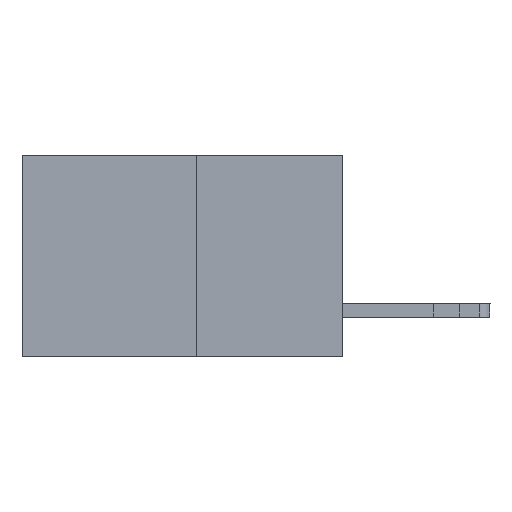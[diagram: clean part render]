
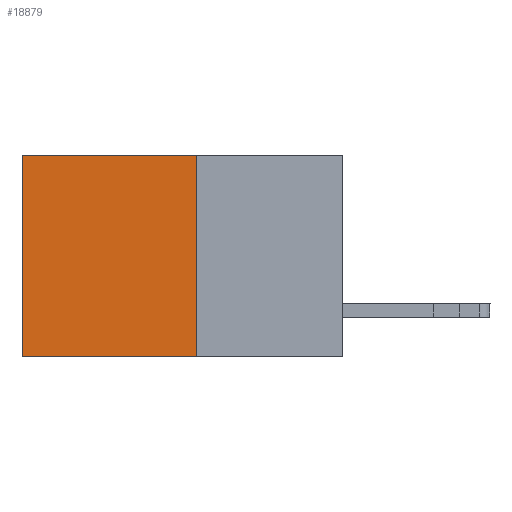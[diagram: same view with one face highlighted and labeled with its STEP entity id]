
A CAD part, left-side view. The second image highlights one B-rep face of the part: STEP entity #18879.
In plain terms, the highlighted planar face has unit normal (-1, 0, 0).
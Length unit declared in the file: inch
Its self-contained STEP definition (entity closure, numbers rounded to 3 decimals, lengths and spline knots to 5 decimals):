
#295 = LINE ( 'NONE', #2195, #8293 ) ;
#578 = VECTOR ( 'NONE', #15893, 39.37008 ) ;
#2097 = EDGE_CURVE ( 'NONE', #9896, #18401, #14686, .T. ) ;
#2195 = CARTESIAN_POINT ( 'NONE',  ( 0.277, 0.27, -0.37 ) ) ;
#2197 = AXIS2_PLACEMENT_3D ( 'NONE', #18991, #5157, #15972 ) ;
#2531 = CARTESIAN_POINT ( 'NONE',  ( 0.277, 0.59, 0. ) ) ;
#3312 = ORIENTED_EDGE ( 'NONE', *, *, #7692, .T. ) ;
#4095 = FACE_OUTER_BOUND ( 'NONE', #8048, .T. ) ;
#4135 = VERTEX_POINT ( 'NONE', #4486 ) ;
#4330 = ORIENTED_EDGE ( 'NONE', *, *, #6906, .F. ) ;
#4404 = CARTESIAN_POINT ( 'NONE',  ( 0.277, 0.59, -0.37 ) ) ;
#4486 = CARTESIAN_POINT ( 'NONE',  ( 0.277, 0.59, -0.37 ) ) ;
#4858 = ORIENTED_EDGE ( 'NONE', *, *, #2097, .T. ) ;
#5157 = DIRECTION ( 'NONE',  ( 1., 0., 0. ) ) ;
#5713 = DIRECTION ( 'NONE',  ( 0., 1., 0. ) ) ;
#6435 = VECTOR ( 'NONE', #5713, 39.37008 ) ;
#6906 = EDGE_CURVE ( 'NONE', #9896, #13718, #295, .T. ) ;
#7692 = EDGE_CURVE ( 'NONE', #18401, #4135, #13363, .T. ) ;
#8048 = EDGE_LOOP ( 'NONE', ( #3312, #8094, #4330, #4858 ) ) ;
#8094 = ORIENTED_EDGE ( 'NONE', *, *, #19465, .F. ) ;
#8293 = VECTOR ( 'NONE', #11755, 39.37008 ) ;
#9080 = LINE ( 'NONE', #18908, #578 ) ;
#9250 = CARTESIAN_POINT ( 'NONE',  ( 0.277, 0.27, 0. ) ) ;
#9896 = VERTEX_POINT ( 'NONE', #16822 ) ;
#11755 = DIRECTION ( 'NONE',  ( 0., 0., -1. ) ) ;
#11830 = CARTESIAN_POINT ( 'NONE',  ( 0.277, 0.27, -0.37 ) ) ;
#12897 = VECTOR ( 'NONE', #16819, 39.37008 ) ;
#13363 = LINE ( 'NONE', #4404, #12897 ) ;
#13718 = VERTEX_POINT ( 'NONE', #11830 ) ;
#14476 = PLANE ( 'NONE',  #2197 ) ;
#14686 = LINE ( 'NONE', #9250, #6435 ) ;
#15893 = DIRECTION ( 'NONE',  ( 0., 1., 0. ) ) ;
#15972 = DIRECTION ( 'NONE',  ( 0., 0., -1. ) ) ;
#16819 = DIRECTION ( 'NONE',  ( 0., 0., -1. ) ) ;
#16822 = CARTESIAN_POINT ( 'NONE',  ( 0.277, 0.27, 0. ) ) ;
#18401 = VERTEX_POINT ( 'NONE', #2531 ) ;
#18879 = ADVANCED_FACE ( 'NONE', ( #4095 ), #14476, .F. ) ;
#18908 = CARTESIAN_POINT ( 'NONE',  ( 0.277, 0.27, -0.37 ) ) ;
#18991 = CARTESIAN_POINT ( 'NONE',  ( 0.277, 0.27, -0.37 ) ) ;
#19465 = EDGE_CURVE ( 'NONE', #13718, #4135, #9080, .T. ) ;
